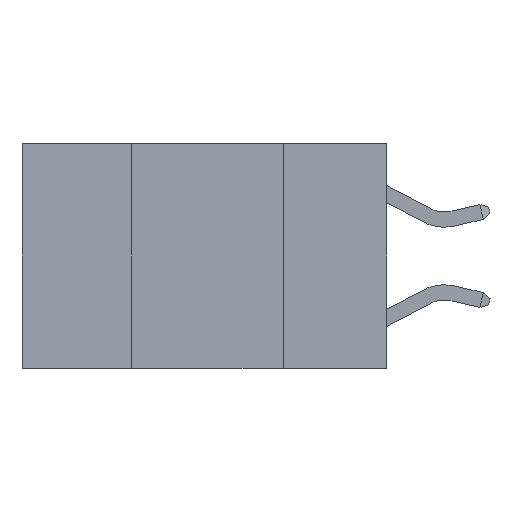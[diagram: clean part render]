
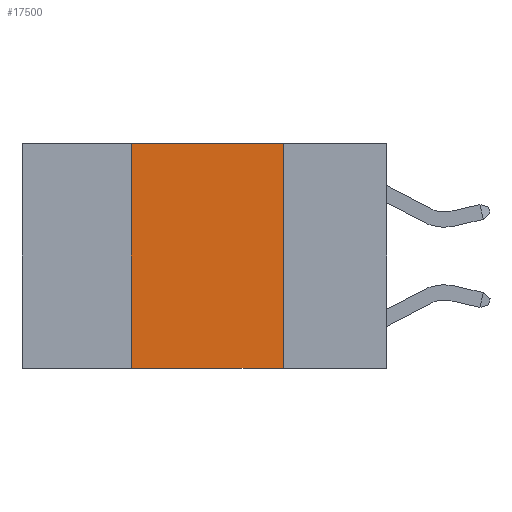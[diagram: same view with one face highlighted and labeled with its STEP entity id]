
A CAD part, left-side view. The second image highlights one B-rep face of the part: STEP entity #17500.
In plain terms, the highlighted planar face has unit normal (-1, 0, 0).
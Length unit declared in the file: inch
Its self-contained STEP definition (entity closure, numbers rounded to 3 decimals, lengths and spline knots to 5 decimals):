
#335 = EDGE_CURVE ( 'NONE', #11549, #570, #3049, .T. ) ;
#570 = VERTEX_POINT ( 'NONE', #11932 ) ;
#1526 = DIRECTION ( 'NONE',  ( 0., -1., 0. ) ) ;
#1963 = CARTESIAN_POINT ( 'NONE',  ( 0., 0.6, 0. ) ) ;
#3049 = LINE ( 'NONE', #9190, #15428 ) ;
#4474 = DIRECTION ( 'NONE',  ( 1., 0., 0. ) ) ;
#4957 = FACE_OUTER_BOUND ( 'NONE', #23852, .T. ) ;
#5377 = EDGE_CURVE ( 'NONE', #13483, #7350, #25446, .T. ) ;
#6124 = LINE ( 'NONE', #31055, #18440 ) ;
#6542 = ORIENTED_EDGE ( 'NONE', *, *, #18818, .T. ) ;
#6695 = CARTESIAN_POINT ( 'NONE',  ( 0., 0.42, -0.37 ) ) ;
#7350 = VERTEX_POINT ( 'NONE', #12437 ) ;
#9190 = CARTESIAN_POINT ( 'NONE',  ( 0., 0.17, 0. ) ) ;
#10858 = VECTOR ( 'NONE', #19311, 39.37008 ) ;
#11360 = ORIENTED_EDGE ( 'NONE', *, *, #335, .F. ) ;
#11549 = VERTEX_POINT ( 'NONE', #27168 ) ;
#11932 = CARTESIAN_POINT ( 'NONE',  ( 0., 0.17, -0.37 ) ) ;
#12140 = DIRECTION ( 'NONE',  ( 0., 0., -1. ) ) ;
#12437 = CARTESIAN_POINT ( 'NONE',  ( 0., 0.42, 0. ) ) ;
#13483 = VERTEX_POINT ( 'NONE', #6695 ) ;
#15428 = VECTOR ( 'NONE', #12140, 39.37008 ) ;
#17420 = ORIENTED_EDGE ( 'NONE', *, *, #5377, .F. ) ;
#17500 = ADVANCED_FACE ( 'NONE', ( #4957 ), #31473, .F. ) ;
#18440 = VECTOR ( 'NONE', #1526, 39.37008 ) ;
#18810 = AXIS2_PLACEMENT_3D ( 'NONE', #1963, #4474, #21708 ) ;
#18818 = EDGE_CURVE ( 'NONE', #13483, #570, #6124, .T. ) ;
#19311 = DIRECTION ( 'NONE',  ( 0., 0., 1. ) ) ;
#20070 = ORIENTED_EDGE ( 'NONE', *, *, #30005, .F. ) ;
#21708 = DIRECTION ( 'NONE',  ( 0., 0., -1. ) ) ;
#21994 = DIRECTION ( 'NONE',  ( 0., -1., 0. ) ) ;
#23852 = EDGE_LOOP ( 'NONE', ( #11360, #20070, #17420, #6542 ) ) ;
#24153 = VECTOR ( 'NONE', #21994, 39.37008 ) ;
#24315 = CARTESIAN_POINT ( 'NONE',  ( 0., 0.6, 0. ) ) ;
#24943 = LINE ( 'NONE', #24315, #24153 ) ;
#25446 = LINE ( 'NONE', #26590, #10858 ) ;
#26590 = CARTESIAN_POINT ( 'NONE',  ( 0., 0.42, 0. ) ) ;
#27168 = CARTESIAN_POINT ( 'NONE',  ( 0., 0.17, 0. ) ) ;
#30005 = EDGE_CURVE ( 'NONE', #7350, #11549, #24943, .T. ) ;
#31055 = CARTESIAN_POINT ( 'NONE',  ( 0., 0.6, -0.37 ) ) ;
#31473 = PLANE ( 'NONE',  #18810 ) ;
